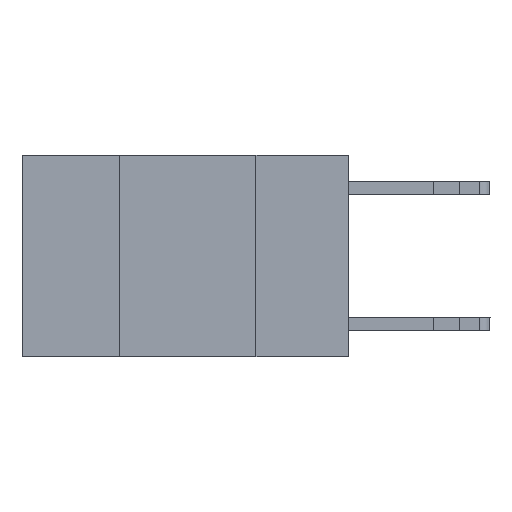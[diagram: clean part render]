
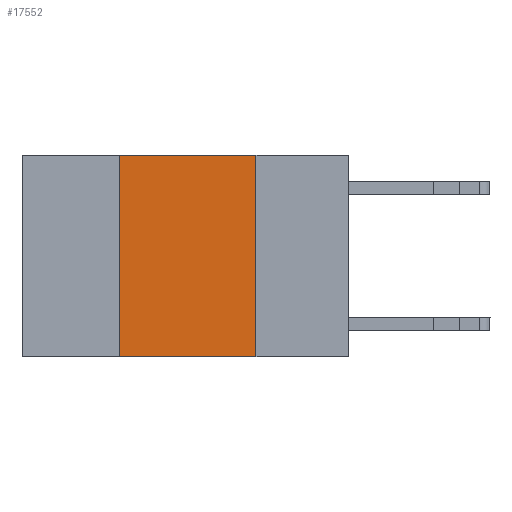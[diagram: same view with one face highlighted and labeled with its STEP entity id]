
A CAD part, left-side view. The second image highlights one B-rep face of the part: STEP entity #17552.
In plain terms, the highlighted planar face has unit normal (-1, 0, 0).
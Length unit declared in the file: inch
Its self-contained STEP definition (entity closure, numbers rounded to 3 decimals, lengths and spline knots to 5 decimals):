
#1893 = CARTESIAN_POINT ( 'NONE',  ( 0., 0.42, 0. ) ) ;
#3602 = VERTEX_POINT ( 'NONE', #1893 ) ;
#4234 = PLANE ( 'NONE',  #27569 ) ;
#4552 = CARTESIAN_POINT ( 'NONE',  ( 0., 0.6, 0. ) ) ;
#7285 = VERTEX_POINT ( 'NONE', #17088 ) ;
#8113 = CARTESIAN_POINT ( 'NONE',  ( 0., 0.42, 0. ) ) ;
#8165 = VECTOR ( 'NONE', #25366, 39.37008 ) ;
#8186 = LINE ( 'NONE', #8113, #8165 ) ;
#8201 = EDGE_CURVE ( 'NONE', #7285, #18677, #17387, .T. ) ;
#8330 = EDGE_CURVE ( 'NONE', #18257, #18677, #15867, .T. ) ;
#8623 = ORIENTED_EDGE ( 'NONE', *, *, #8330, .F. ) ;
#8735 = ORIENTED_EDGE ( 'NONE', *, *, #24705, .F. ) ;
#8883 = ORIENTED_EDGE ( 'NONE', *, *, #13434, .F. ) ;
#9137 = FACE_OUTER_BOUND ( 'NONE', #21710, .T. ) ;
#9288 = ORIENTED_EDGE ( 'NONE', *, *, #8201, .T. ) ;
#10960 = DIRECTION ( 'NONE',  ( 1., 0., 0. ) ) ;
#11501 = CARTESIAN_POINT ( 'NONE',  ( 0., 0.17, 0. ) ) ;
#12791 = CARTESIAN_POINT ( 'NONE',  ( 0., 0.17, -0.37 ) ) ;
#13434 = EDGE_CURVE ( 'NONE', #7285, #3602, #8186, .T. ) ;
#14756 = LINE ( 'NONE', #4552, #26759 ) ;
#15042 = DIRECTION ( 'NONE',  ( 0., -1., 0. ) ) ;
#15753 = VECTOR ( 'NONE', #19707, 39.37008 ) ;
#15867 = LINE ( 'NONE', #21763, #15753 ) ;
#16872 = VECTOR ( 'NONE', #15042, 39.37008 ) ;
#17088 = CARTESIAN_POINT ( 'NONE',  ( 0., 0.42, -0.37 ) ) ;
#17387 = LINE ( 'NONE', #23545, #16872 ) ;
#17552 = ADVANCED_FACE ( 'NONE', ( #9137 ), #4234, .F. ) ;
#18257 = VERTEX_POINT ( 'NONE', #11501 ) ;
#18677 = VERTEX_POINT ( 'NONE', #12791 ) ;
#19531 = CARTESIAN_POINT ( 'NONE',  ( 0., 0.6, 0. ) ) ;
#19707 = DIRECTION ( 'NONE',  ( 0., 0., -1. ) ) ;
#21710 = EDGE_LOOP ( 'NONE', ( #8623, #8735, #8883, #9288 ) ) ;
#21763 = CARTESIAN_POINT ( 'NONE',  ( 0., 0.17, 0. ) ) ;
#23545 = CARTESIAN_POINT ( 'NONE',  ( 0., 0.6, -0.37 ) ) ;
#24120 = DIRECTION ( 'NONE',  ( 0., -1., 0. ) ) ;
#24705 = EDGE_CURVE ( 'NONE', #3602, #18257, #14756, .T. ) ;
#25366 = DIRECTION ( 'NONE',  ( 0., 0., 1. ) ) ;
#25939 = DIRECTION ( 'NONE',  ( 0., 0., -1. ) ) ;
#26759 = VECTOR ( 'NONE', #24120, 39.37008 ) ;
#27569 = AXIS2_PLACEMENT_3D ( 'NONE', #19531, #10960, #25939 ) ;
